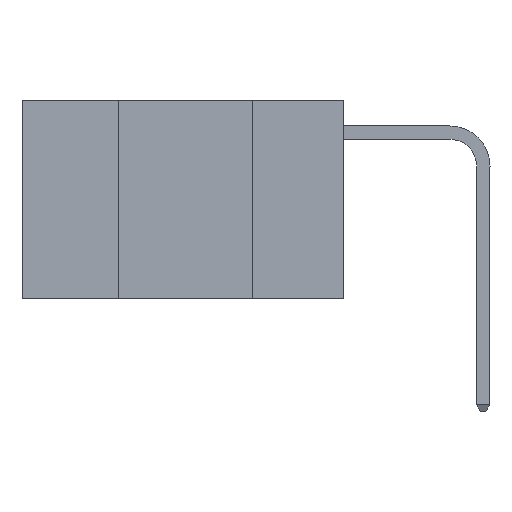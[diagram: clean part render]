
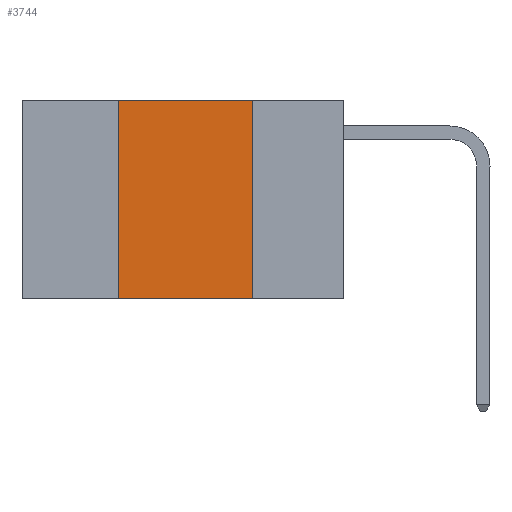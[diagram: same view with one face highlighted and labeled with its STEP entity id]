
A CAD part, left-side view. The second image highlights one B-rep face of the part: STEP entity #3744.
In plain terms, the highlighted planar face has unit normal (-1, 0, 0).
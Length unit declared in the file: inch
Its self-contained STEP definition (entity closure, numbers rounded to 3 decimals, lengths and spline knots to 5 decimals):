
#353 = CARTESIAN_POINT ( 'NONE',  ( 0., 0.17, 0. ) ) ;
#1527 = CARTESIAN_POINT ( 'NONE',  ( 0., 0.17, 0. ) ) ;
#1729 = VERTEX_POINT ( 'NONE', #22861 ) ;
#3744 = ADVANCED_FACE ( 'NONE', ( #14940 ), #5924, .F. ) ;
#3838 = CARTESIAN_POINT ( 'NONE',  ( 0., 0.17, -0.37 ) ) ;
#4657 = EDGE_CURVE ( 'NONE', #1729, #9716, #20366, .T. ) ;
#5374 = EDGE_CURVE ( 'NONE', #5921, #1729, #24683, .T. ) ;
#5520 = DIRECTION ( 'NONE',  ( 0., 0., -1. ) ) ;
#5634 = ORIENTED_EDGE ( 'NONE', *, *, #6758, .F. ) ;
#5921 = VERTEX_POINT ( 'NONE', #15539 ) ;
#5924 = PLANE ( 'NONE',  #10761 ) ;
#6591 = VECTOR ( 'NONE', #19906, 39.37008 ) ;
#6758 = EDGE_CURVE ( 'NONE', #9716, #13256, #12038, .T. ) ;
#6905 = ORIENTED_EDGE ( 'NONE', *, *, #8126, .T. ) ;
#7644 = CARTESIAN_POINT ( 'NONE',  ( 0., 0.42, 0. ) ) ;
#8080 = ORIENTED_EDGE ( 'NONE', *, *, #4657, .F. ) ;
#8126 = EDGE_CURVE ( 'NONE', #5921, #13256, #22673, .T. ) ;
#8452 = DIRECTION ( 'NONE',  ( 1., 0., 0. ) ) ;
#9716 = VERTEX_POINT ( 'NONE', #353 ) ;
#10184 = EDGE_LOOP ( 'NONE', ( #5634, #8080, #11281, #6905 ) ) ;
#10761 = AXIS2_PLACEMENT_3D ( 'NONE', #20141, #8452, #5520 ) ;
#11243 = CARTESIAN_POINT ( 'NONE',  ( 0., 0.6, 0. ) ) ;
#11281 = ORIENTED_EDGE ( 'NONE', *, *, #5374, .F. ) ;
#12038 = LINE ( 'NONE', #1527, #6591 ) ;
#13256 = VERTEX_POINT ( 'NONE', #3838 ) ;
#13333 = DIRECTION ( 'NONE',  ( 0., -1., 0. ) ) ;
#13595 = CARTESIAN_POINT ( 'NONE',  ( 0., 0.6, -0.37 ) ) ;
#13689 = DIRECTION ( 'NONE',  ( 0., -1., 0. ) ) ;
#13857 = DIRECTION ( 'NONE',  ( 0., 0., 1. ) ) ;
#14940 = FACE_OUTER_BOUND ( 'NONE', #10184, .T. ) ;
#15085 = VECTOR ( 'NONE', #13333, 39.37008 ) ;
#15539 = CARTESIAN_POINT ( 'NONE',  ( 0., 0.42, -0.37 ) ) ;
#16755 = VECTOR ( 'NONE', #13689, 39.37008 ) ;
#19382 = VECTOR ( 'NONE', #13857, 39.37008 ) ;
#19906 = DIRECTION ( 'NONE',  ( 0., 0., -1. ) ) ;
#20141 = CARTESIAN_POINT ( 'NONE',  ( 0., 0.6, 0. ) ) ;
#20366 = LINE ( 'NONE', #11243, #15085 ) ;
#22673 = LINE ( 'NONE', #13595, #16755 ) ;
#22861 = CARTESIAN_POINT ( 'NONE',  ( 0., 0.42, 0. ) ) ;
#24683 = LINE ( 'NONE', #7644, #19382 ) ;
